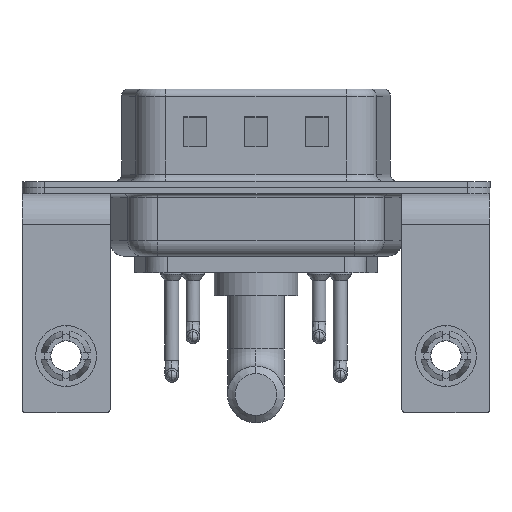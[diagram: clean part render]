
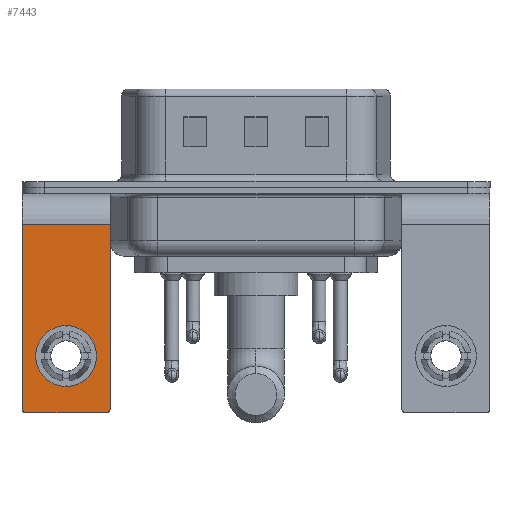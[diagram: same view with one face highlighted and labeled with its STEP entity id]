
A CAD part, front view. The second image highlights one B-rep face of the part: STEP entity #7443.
In plain terms, the highlighted planar face has unit normal (0, -1, 0).
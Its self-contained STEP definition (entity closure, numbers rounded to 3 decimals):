
#195 = VERTEX_POINT ( 'NONE', #4607 ) ;
#233 = CARTESIAN_POINT ( 'NONE',  ( 2.9, -6.25, -14.8 ) ) ;
#883 = VECTOR ( 'NONE', #17565, 1000. ) ;
#1008 = CARTESIAN_POINT ( 'NONE',  ( -2.9, -6.25, -14.55 ) ) ;
#1145 = CARTESIAN_POINT ( 'NONE',  ( 2.9, -6.25, -2.4 ) ) ;
#1385 = VERTEX_POINT ( 'NONE', #17768 ) ;
#1795 = DIRECTION ( 'NONE',  ( 0., 0., 1. ) ) ;
#2027 = VERTEX_POINT ( 'NONE', #20337 ) ;
#2269 = EDGE_CURVE ( 'NONE', #11409, #1385, #4214, .T. ) ;
#2516 = LINE ( 'NONE', #16019, #883 ) ;
#2678 = LINE ( 'NONE', #8940, #15198 ) ;
#2795 = DIRECTION ( 'NONE',  ( 0., 1., 0. ) ) ;
#3156 = AXIS2_PLACEMENT_3D ( 'NONE', #12886, #4984, #8054 ) ;
#3280 = CIRCLE ( 'NONE', #21161, 2. ) ;
#3896 = LINE ( 'NONE', #20899, #16548 ) ;
#4214 = CIRCLE ( 'NONE', #3156, 0.25 ) ;
#4607 = CARTESIAN_POINT ( 'NONE',  ( 0., -6.25, -9.07 ) ) ;
#4668 = CARTESIAN_POINT ( 'NONE',  ( 2.9, -6.25, -2.4 ) ) ;
#4681 = CARTESIAN_POINT ( 'NONE',  ( 0., -6.25, -11.07 ) ) ;
#4918 = VERTEX_POINT ( 'NONE', #20140 ) ;
#4984 = DIRECTION ( 'NONE',  ( 0., -1., 0. ) ) ;
#4985 = DIRECTION ( 'NONE',  ( 0., 0., 1. ) ) ;
#5070 = ORIENTED_EDGE ( 'NONE', *, *, #6439, .F. ) ;
#5212 = CIRCLE ( 'NONE', #17470, 0.25 ) ;
#5604 = EDGE_CURVE ( 'NONE', #10863, #21266, #2516, .T. ) ;
#6439 = EDGE_CURVE ( 'NONE', #13714, #1385, #15283, .T. ) ;
#6493 = DIRECTION ( 'NONE',  ( 0., 0., 1. ) ) ;
#7443 = ADVANCED_FACE ( 'NONE', ( #8055, #14857 ), #16730, .F. ) ;
#7620 = ORIENTED_EDGE ( 'NONE', *, *, #5604, .T. ) ;
#8054 = DIRECTION ( 'NONE',  ( 0., 0., 1. ) ) ;
#8055 = FACE_BOUND ( 'NONE', #18297, .T. ) ;
#8940 = CARTESIAN_POINT ( 'NONE',  ( 2.9, -6.25, -2.4 ) ) ;
#9270 = ORIENTED_EDGE ( 'NONE', *, *, #19178, .F. ) ;
#9286 = EDGE_CURVE ( 'NONE', #13714, #2027, #5212, .T. ) ;
#9492 = DIRECTION ( 'NONE',  ( 0., 0., 1. ) ) ;
#10863 = VERTEX_POINT ( 'NONE', #1145 ) ;
#11277 = ORIENTED_EDGE ( 'NONE', *, *, #20847, .T. ) ;
#11409 = VERTEX_POINT ( 'NONE', #1008 ) ;
#11460 = VECTOR ( 'NONE', #11987, 1000. ) ;
#11987 = DIRECTION ( 'NONE',  ( -1., 0., 0. ) ) ;
#12308 = EDGE_CURVE ( 'NONE', #195, #4918, #18981, .T. ) ;
#12451 = DIRECTION ( 'NONE',  ( 0., 0., -1. ) ) ;
#12886 = CARTESIAN_POINT ( 'NONE',  ( -2.65, -6.25, -14.55 ) ) ;
#13085 = CARTESIAN_POINT ( 'NONE',  ( 2.65, -6.25, -14.55 ) ) ;
#13544 = DIRECTION ( 'NONE',  ( 0., 1., 0. ) ) ;
#13714 = VERTEX_POINT ( 'NONE', #16857 ) ;
#14734 = CARTESIAN_POINT ( 'NONE',  ( -2.9, -6.25, -2.4 ) ) ;
#14857 = FACE_OUTER_BOUND ( 'NONE', #21157, .T. ) ;
#15125 = ORIENTED_EDGE ( 'NONE', *, *, #9286, .T. ) ;
#15198 = VECTOR ( 'NONE', #12451, 1000. ) ;
#15283 = LINE ( 'NONE', #233, #11460 ) ;
#16019 = CARTESIAN_POINT ( 'NONE',  ( 2.9, -6.25, -2.4 ) ) ;
#16548 = VECTOR ( 'NONE', #20685, 1000. ) ;
#16730 = PLANE ( 'NONE',  #20587 ) ;
#16857 = CARTESIAN_POINT ( 'NONE',  ( 2.65, -6.25, -14.8 ) ) ;
#17470 = AXIS2_PLACEMENT_3D ( 'NONE', #13085, #21539, #6493 ) ;
#17565 = DIRECTION ( 'NONE',  ( -1., 0., 0. ) ) ;
#17768 = CARTESIAN_POINT ( 'NONE',  ( -2.65, -6.25, -14.8 ) ) ;
#17860 = ORIENTED_EDGE ( 'NONE', *, *, #12308, .T. ) ;
#17955 = EDGE_CURVE ( 'NONE', #21266, #11409, #3896, .T. ) ;
#18028 = ORIENTED_EDGE ( 'NONE', *, *, #2269, .T. ) ;
#18274 = AXIS2_PLACEMENT_3D ( 'NONE', #4681, #2795, #9492 ) ;
#18297 = EDGE_LOOP ( 'NONE', ( #11277, #17860 ) ) ;
#18981 = CIRCLE ( 'NONE', #18274, 2. ) ;
#19178 = EDGE_CURVE ( 'NONE', #10863, #2027, #2678, .T. ) ;
#19585 = DIRECTION ( 'NONE',  ( 0., 1., 0. ) ) ;
#20140 = CARTESIAN_POINT ( 'NONE',  ( 0., -6.25, -13.07 ) ) ;
#20337 = CARTESIAN_POINT ( 'NONE',  ( 2.9, -6.25, -14.55 ) ) ;
#20351 = ORIENTED_EDGE ( 'NONE', *, *, #17955, .T. ) ;
#20561 = CARTESIAN_POINT ( 'NONE',  ( 0., -6.25, -11.07 ) ) ;
#20587 = AXIS2_PLACEMENT_3D ( 'NONE', #4668, #19585, #4985 ) ;
#20685 = DIRECTION ( 'NONE',  ( 0., 0., -1. ) ) ;
#20847 = EDGE_CURVE ( 'NONE', #4918, #195, #3280, .T. ) ;
#20899 = CARTESIAN_POINT ( 'NONE',  ( -2.9, -6.25, -2.4 ) ) ;
#21157 = EDGE_LOOP ( 'NONE', ( #20351, #18028, #5070, #15125, #9270, #7620 ) ) ;
#21161 = AXIS2_PLACEMENT_3D ( 'NONE', #20561, #13544, #1795 ) ;
#21266 = VERTEX_POINT ( 'NONE', #14734 ) ;
#21539 = DIRECTION ( 'NONE',  ( 0., -1., 0. ) ) ;
